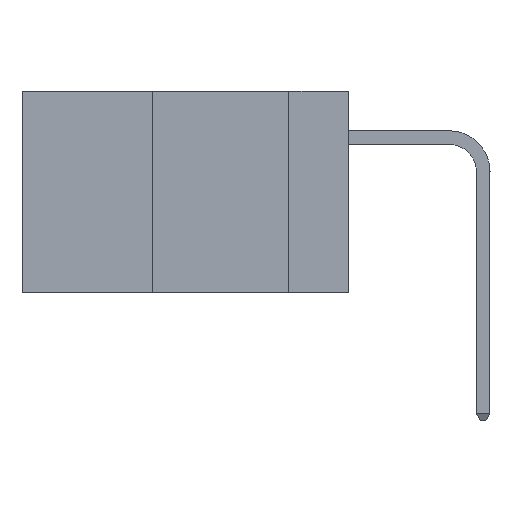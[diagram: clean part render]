
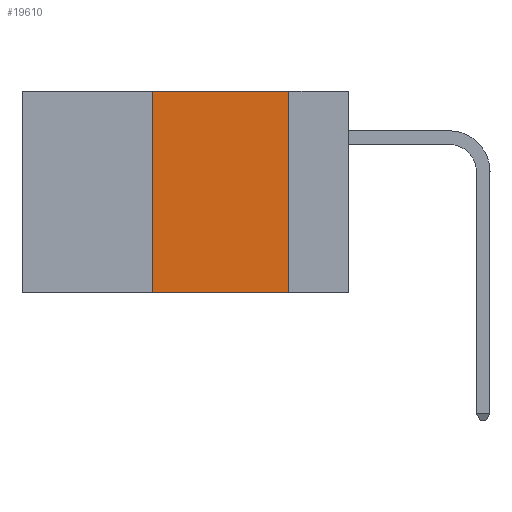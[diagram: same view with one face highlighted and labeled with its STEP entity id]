
A CAD part, left-side view. The second image highlights one B-rep face of the part: STEP entity #19610.
In plain terms, the highlighted planar face has unit normal (-1, 0, 0).
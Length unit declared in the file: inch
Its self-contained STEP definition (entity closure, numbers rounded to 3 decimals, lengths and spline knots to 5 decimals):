
#741 = FACE_OUTER_BOUND ( 'NONE', #35894, .T. ) ;
#1991 = DIRECTION ( 'NONE',  ( 0., 0., -1. ) ) ;
#4009 = VECTOR ( 'NONE', #6123, 39.37008 ) ;
#4767 = ORIENTED_EDGE ( 'NONE', *, *, #19760, .F. ) ;
#6123 = DIRECTION ( 'NONE',  ( 0., 0., -1. ) ) ;
#6760 = EDGE_CURVE ( 'NONE', #30778, #12373, #27248, .T. ) ;
#7677 = CARTESIAN_POINT ( 'NONE',  ( 0., 0.36, 0. ) ) ;
#8165 = CARTESIAN_POINT ( 'NONE',  ( 0., 0.11, 0. ) ) ;
#8406 = CARTESIAN_POINT ( 'NONE',  ( 0., 0.36, 0. ) ) ;
#8971 = ORIENTED_EDGE ( 'NONE', *, *, #28154, .T. ) ;
#9079 = CARTESIAN_POINT ( 'NONE',  ( 0., 0.11, 0. ) ) ;
#11510 = DIRECTION ( 'NONE',  ( 0., -1., 0. ) ) ;
#12373 = VERTEX_POINT ( 'NONE', #25095 ) ;
#12556 = VERTEX_POINT ( 'NONE', #8406 ) ;
#12575 = VECTOR ( 'NONE', #22252, 39.37008 ) ;
#15937 = LINE ( 'NONE', #28846, #23628 ) ;
#16661 = CARTESIAN_POINT ( 'NONE',  ( 0., 0.6, 0. ) ) ;
#19606 = DIRECTION ( 'NONE',  ( 1., 0., 0. ) ) ;
#19610 = ADVANCED_FACE ( 'NONE', ( #741 ), #33878, .F. ) ;
#19760 = EDGE_CURVE ( 'NONE', #12556, #30778, #15937, .T. ) ;
#22252 = DIRECTION ( 'NONE',  ( 0., 0., 1. ) ) ;
#22990 = VERTEX_POINT ( 'NONE', #26141 ) ;
#23137 = LINE ( 'NONE', #33983, #30707 ) ;
#23628 = VECTOR ( 'NONE', #11510, 39.37008 ) ;
#24370 = ORIENTED_EDGE ( 'NONE', *, *, #6760, .F. ) ;
#25095 = CARTESIAN_POINT ( 'NONE',  ( 0., 0.11, -0.37 ) ) ;
#25315 = DIRECTION ( 'NONE',  ( 0., -1., 0. ) ) ;
#26141 = CARTESIAN_POINT ( 'NONE',  ( 0., 0.36, -0.37 ) ) ;
#27248 = LINE ( 'NONE', #9079, #4009 ) ;
#28154 = EDGE_CURVE ( 'NONE', #22990, #12373, #23137, .T. ) ;
#28403 = AXIS2_PLACEMENT_3D ( 'NONE', #16661, #19606, #1991 ) ;
#28846 = CARTESIAN_POINT ( 'NONE',  ( 0., 0.6, 0. ) ) ;
#30707 = VECTOR ( 'NONE', #25315, 39.37008 ) ;
#30778 = VERTEX_POINT ( 'NONE', #8165 ) ;
#33878 = PLANE ( 'NONE',  #28403 ) ;
#33983 = CARTESIAN_POINT ( 'NONE',  ( 0., 0.6, -0.37 ) ) ;
#34291 = ORIENTED_EDGE ( 'NONE', *, *, #34664, .F. ) ;
#34664 = EDGE_CURVE ( 'NONE', #22990, #12556, #35585, .T. ) ;
#35585 = LINE ( 'NONE', #7677, #12575 ) ;
#35894 = EDGE_LOOP ( 'NONE', ( #24370, #4767, #34291, #8971 ) ) ;
